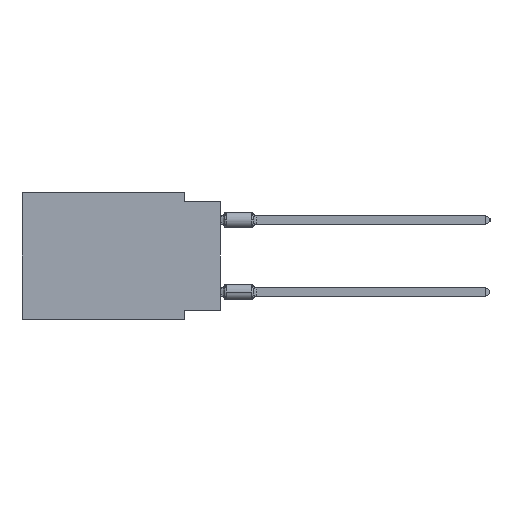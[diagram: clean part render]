
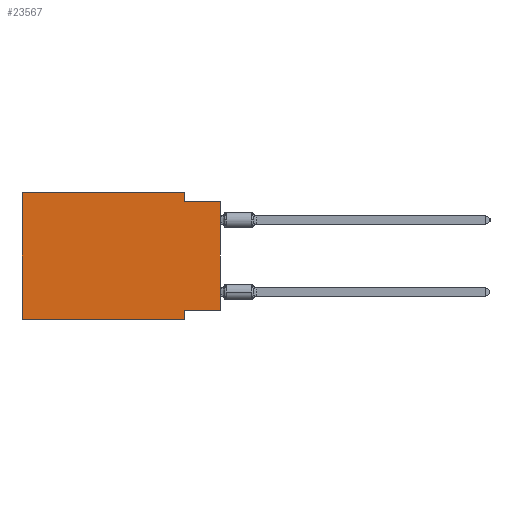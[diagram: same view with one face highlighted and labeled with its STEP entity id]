
A CAD part, left-side view. The second image highlights one B-rep face of the part: STEP entity #23567.
In plain terms, the highlighted planar face has unit normal (-1, 0, 0).
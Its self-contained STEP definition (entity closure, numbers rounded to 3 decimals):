
#163 = VERTEX_POINT ( 'NONE', #21278 ) ;
#409 = EDGE_CURVE ( 'NONE', #4118, #7469, #20914, .T. ) ;
#949 = ORIENTED_EDGE ( 'NONE', *, *, #26595, .F. ) ;
#1246 = VECTOR ( 'NONE', #15158, 1000. ) ;
#1489 = CARTESIAN_POINT ( 'NONE',  ( 0., 0., -8.255 ) ) ;
#1915 = DIRECTION ( 'NONE',  ( 0., -1., 0. ) ) ;
#1936 = CARTESIAN_POINT ( 'NONE',  ( 0., 2.54, -8.89 ) ) ;
#2249 = CARTESIAN_POINT ( 'NONE',  ( 0., 0., -0.635 ) ) ;
#2376 = VERTEX_POINT ( 'NONE', #13088 ) ;
#2494 = AXIS2_PLACEMENT_3D ( 'NONE', #31602, #26139, #4108 ) ;
#3342 = VECTOR ( 'NONE', #16405, 1000. ) ;
#3961 = CARTESIAN_POINT ( 'NONE',  ( 0., 0., -0.635 ) ) ;
#4108 = DIRECTION ( 'NONE',  ( 0., 0., -1. ) ) ;
#4118 = VERTEX_POINT ( 'NONE', #18106 ) ;
#5048 = VERTEX_POINT ( 'NONE', #21150 ) ;
#5895 = LINE ( 'NONE', #15006, #1246 ) ;
#7028 = VECTOR ( 'NONE', #9504, 1000. ) ;
#7228 = CARTESIAN_POINT ( 'NONE',  ( 0., 2.54, -8.89 ) ) ;
#7469 = VERTEX_POINT ( 'NONE', #26499 ) ;
#7989 = EDGE_CURVE ( 'NONE', #17102, #4118, #5895, .T. ) ;
#9504 = DIRECTION ( 'NONE',  ( 0., 0., -1. ) ) ;
#9516 = VERTEX_POINT ( 'NONE', #3961 ) ;
#11424 = VECTOR ( 'NONE', #1915, 1000. ) ;
#12101 = CARTESIAN_POINT ( 'NONE',  ( 0., 13.97, -8.89 ) ) ;
#12553 = DIRECTION ( 'NONE',  ( 0., 0., 1. ) ) ;
#13088 = CARTESIAN_POINT ( 'NONE',  ( 0., 0., -8.255 ) ) ;
#13153 = CARTESIAN_POINT ( 'NONE',  ( 0., 2.54, 0. ) ) ;
#13159 = VECTOR ( 'NONE', #31452, 1000. ) ;
#14427 = CARTESIAN_POINT ( 'NONE',  ( 0., 13.97, -8.89 ) ) ;
#15006 = CARTESIAN_POINT ( 'NONE',  ( 0., 13.97, 0. ) ) ;
#15158 = DIRECTION ( 'NONE',  ( 0., 0., 1. ) ) ;
#15439 = ORIENTED_EDGE ( 'NONE', *, *, #409, .F. ) ;
#15938 = LINE ( 'NONE', #27682, #24054 ) ;
#16143 = EDGE_CURVE ( 'NONE', #2376, #5048, #29466, .T. ) ;
#16405 = DIRECTION ( 'NONE',  ( 0., -1., 0. ) ) ;
#16426 = VECTOR ( 'NONE', #30790, 1000. ) ;
#17102 = VERTEX_POINT ( 'NONE', #12101 ) ;
#17668 = ORIENTED_EDGE ( 'NONE', *, *, #21864, .T. ) ;
#18106 = CARTESIAN_POINT ( 'NONE',  ( 0., 13.97, 0. ) ) ;
#20099 = LINE ( 'NONE', #13153, #30966 ) ;
#20914 = LINE ( 'NONE', #25518, #16426 ) ;
#21150 = CARTESIAN_POINT ( 'NONE',  ( 0., 2.54, -8.255 ) ) ;
#21278 = CARTESIAN_POINT ( 'NONE',  ( 0., 2.54, -0.635 ) ) ;
#21864 = EDGE_CURVE ( 'NONE', #17102, #24913, #21992, .T. ) ;
#21992 = LINE ( 'NONE', #14427, #3342 ) ;
#23199 = DIRECTION ( 'NONE',  ( 0., 0., -1. ) ) ;
#23510 = PLANE ( 'NONE',  #2494 ) ;
#23567 = ADVANCED_FACE ( 'NONE', ( #23675 ), #23510, .F. ) ;
#23675 = FACE_OUTER_BOUND ( 'NONE', #26358, .T. ) ;
#23973 = ORIENTED_EDGE ( 'NONE', *, *, #29140, .T. ) ;
#24054 = VECTOR ( 'NONE', #12553, 1000. ) ;
#24220 = ORIENTED_EDGE ( 'NONE', *, *, #28618, .F. ) ;
#24627 = LINE ( 'NONE', #1936, #7028 ) ;
#24771 = LINE ( 'NONE', #2249, #11424 ) ;
#24799 = ORIENTED_EDGE ( 'NONE', *, *, #7989, .F. ) ;
#24913 = VERTEX_POINT ( 'NONE', #7228 ) ;
#25477 = ORIENTED_EDGE ( 'NONE', *, *, #16143, .F. ) ;
#25518 = CARTESIAN_POINT ( 'NONE',  ( 0., 13.97, 0. ) ) ;
#26139 = DIRECTION ( 'NONE',  ( 1., 0., 0. ) ) ;
#26358 = EDGE_LOOP ( 'NONE', ( #23973, #24220, #30662, #15439, #24799, #17668, #949, #25477 ) ) ;
#26499 = CARTESIAN_POINT ( 'NONE',  ( 0., 2.54, 0. ) ) ;
#26595 = EDGE_CURVE ( 'NONE', #5048, #24913, #24627, .T. ) ;
#27682 = CARTESIAN_POINT ( 'NONE',  ( 0., 0., 0. ) ) ;
#28618 = EDGE_CURVE ( 'NONE', #163, #9516, #24771, .T. ) ;
#29140 = EDGE_CURVE ( 'NONE', #2376, #9516, #15938, .T. ) ;
#29466 = LINE ( 'NONE', #1489, #13159 ) ;
#30662 = ORIENTED_EDGE ( 'NONE', *, *, #30676, .F. ) ;
#30676 = EDGE_CURVE ( 'NONE', #7469, #163, #20099, .T. ) ;
#30790 = DIRECTION ( 'NONE',  ( 0., -1., 0. ) ) ;
#30966 = VECTOR ( 'NONE', #23199, 1000. ) ;
#31452 = DIRECTION ( 'NONE',  ( 0., 1., 0. ) ) ;
#31602 = CARTESIAN_POINT ( 'NONE',  ( 0., 13.97, 0. ) ) ;
